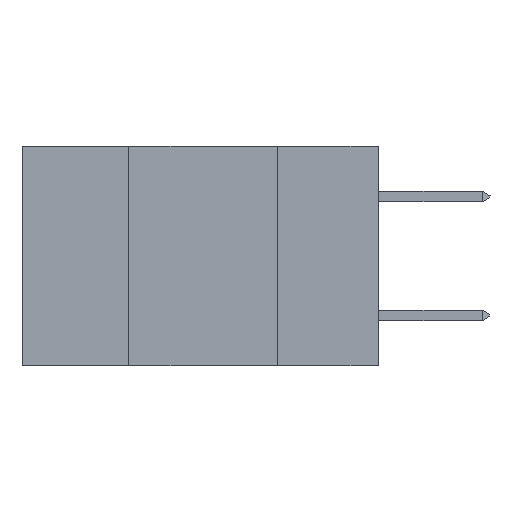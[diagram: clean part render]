
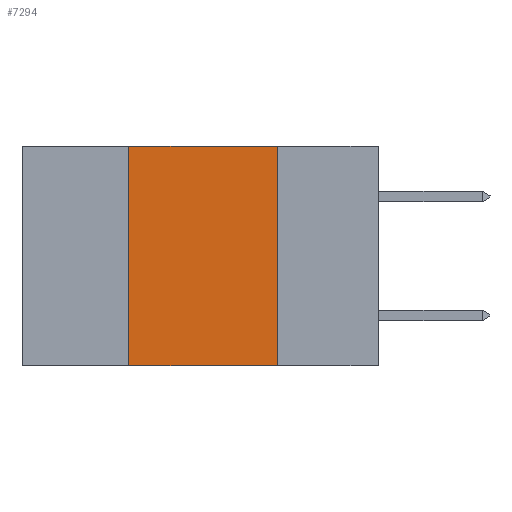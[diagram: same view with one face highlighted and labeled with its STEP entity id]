
A CAD part, left-side view. The second image highlights one B-rep face of the part: STEP entity #7294.
In plain terms, the highlighted planar face has unit normal (-1, 0, 0).
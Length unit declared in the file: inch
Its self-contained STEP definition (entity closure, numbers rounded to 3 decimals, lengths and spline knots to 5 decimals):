
#84 = LINE ( 'NONE', #4547, #3489 ) ;
#422 = CARTESIAN_POINT ( 'NONE',  ( 0., 0.17, 0. ) ) ;
#1229 = CARTESIAN_POINT ( 'NONE',  ( 0., 0.17, -0.37 ) ) ;
#1815 = EDGE_CURVE ( 'NONE', #12253, #3097, #2074, .T. ) ;
#2074 = LINE ( 'NONE', #15203, #11687 ) ;
#2224 = DIRECTION ( 'NONE',  ( 0., 0., -1. ) ) ;
#3097 = VERTEX_POINT ( 'NONE', #422 ) ;
#3224 = LINE ( 'NONE', #12099, #8962 ) ;
#3377 = CARTESIAN_POINT ( 'NONE',  ( 0., 0.17, -0.37 ) ) ;
#3489 = VECTOR ( 'NONE', #6269, 39.37008 ) ;
#3714 = ORIENTED_EDGE ( 'NONE', *, *, #1815, .F. ) ;
#3725 = FACE_OUTER_BOUND ( 'NONE', #10493, .T. ) ;
#4547 = CARTESIAN_POINT ( 'NONE',  ( 0., 0.42, -0.37 ) ) ;
#4984 = VERTEX_POINT ( 'NONE', #1229 ) ;
#5278 = CARTESIAN_POINT ( 'NONE',  ( 0., 0.6, 0. ) ) ;
#6269 = DIRECTION ( 'NONE',  ( 0., 0., 1. ) ) ;
#6470 = LINE ( 'NONE', #3377, #15073 ) ;
#6967 = ORIENTED_EDGE ( 'NONE', *, *, #18691, .F. ) ;
#7294 = ADVANCED_FACE ( 'NONE', ( #3725 ), #18500, .F. ) ;
#7756 = VERTEX_POINT ( 'NONE', #9933 ) ;
#8507 = DIRECTION ( 'NONE',  ( 1., 0., 0. ) ) ;
#8932 = EDGE_CURVE ( 'NONE', #7756, #4984, #3224, .T. ) ;
#8962 = VECTOR ( 'NONE', #15084, 39.37008 ) ;
#9933 = CARTESIAN_POINT ( 'NONE',  ( 0., 0.42, -0.37 ) ) ;
#10493 = EDGE_LOOP ( 'NONE', ( #6967, #3714, #13214, #14292 ) ) ;
#11687 = VECTOR ( 'NONE', #12399, 39.37008 ) ;
#12099 = CARTESIAN_POINT ( 'NONE',  ( 0., 0.6, -0.37 ) ) ;
#12253 = VERTEX_POINT ( 'NONE', #14291 ) ;
#12399 = DIRECTION ( 'NONE',  ( 0., -1., 0. ) ) ;
#12495 = DIRECTION ( 'NONE',  ( 0., 0., -1. ) ) ;
#13214 = ORIENTED_EDGE ( 'NONE', *, *, #14223, .F. ) ;
#14223 = EDGE_CURVE ( 'NONE', #7756, #12253, #84, .T. ) ;
#14291 = CARTESIAN_POINT ( 'NONE',  ( 0., 0.42, 0. ) ) ;
#14292 = ORIENTED_EDGE ( 'NONE', *, *, #8932, .T. ) ;
#15073 = VECTOR ( 'NONE', #2224, 39.37008 ) ;
#15084 = DIRECTION ( 'NONE',  ( 0., -1., 0. ) ) ;
#15203 = CARTESIAN_POINT ( 'NONE',  ( 0., 0.6, 0. ) ) ;
#17109 = AXIS2_PLACEMENT_3D ( 'NONE', #5278, #8507, #12495 ) ;
#18500 = PLANE ( 'NONE',  #17109 ) ;
#18691 = EDGE_CURVE ( 'NONE', #3097, #4984, #6470, .T. ) ;
